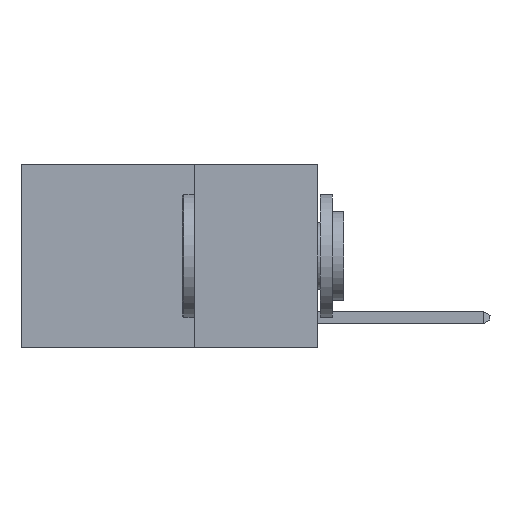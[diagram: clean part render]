
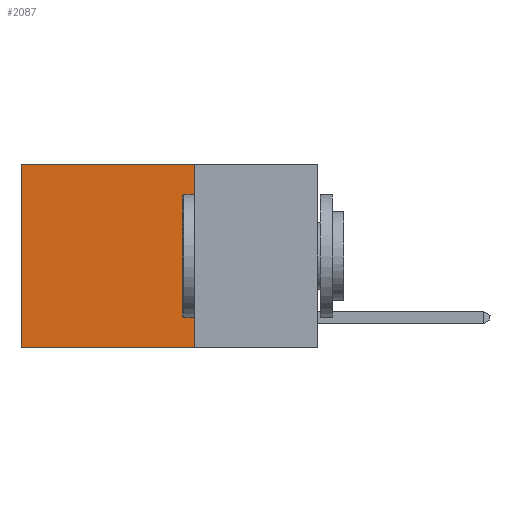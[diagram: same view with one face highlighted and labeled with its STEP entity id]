
A CAD part, left-side view. The second image highlights one B-rep face of the part: STEP entity #2087.
In plain terms, the highlighted planar face has unit normal (-1, 0, 0).
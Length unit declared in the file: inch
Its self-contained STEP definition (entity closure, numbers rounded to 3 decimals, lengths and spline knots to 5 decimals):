
#336 = EDGE_CURVE ( 'NONE', #4194, #12031, #13688, .T. ) ;
#573 = CARTESIAN_POINT ( 'NONE',  ( 0.2625, 0.6, 0. ) ) ;
#1482 = LINE ( 'NONE', #6404, #11278 ) ;
#1989 = VERTEX_POINT ( 'NONE', #8276 ) ;
#1996 = EDGE_CURVE ( 'NONE', #1989, #13666, #3204, .T. ) ;
#2087 = ADVANCED_FACE ( 'NONE', ( #5139 ), #3523, .F. ) ;
#2537 = VECTOR ( 'NONE', #7542, 39.37008 ) ;
#3204 = LINE ( 'NONE', #5644, #10374 ) ;
#3414 = CARTESIAN_POINT ( 'NONE',  ( 0.2625, 0.6, 0. ) ) ;
#3523 = PLANE ( 'NONE',  #10117 ) ;
#3543 = DIRECTION ( 'NONE',  ( 0., 1., 0. ) ) ;
#3694 = CARTESIAN_POINT ( 'NONE',  ( 0.2625, 0.25, 0. ) ) ;
#3885 = EDGE_LOOP ( 'NONE', ( #9423, #12779, #8823, #8395 ) ) ;
#4194 = VERTEX_POINT ( 'NONE', #3414 ) ;
#5139 = FACE_OUTER_BOUND ( 'NONE', #3885, .T. ) ;
#5644 = CARTESIAN_POINT ( 'NONE',  ( 0.2625, 0.25, 0. ) ) ;
#5944 = DIRECTION ( 'NONE',  ( 0., 0., -1. ) ) ;
#6336 = DIRECTION ( 'NONE',  ( 1., 0., 0. ) ) ;
#6404 = CARTESIAN_POINT ( 'NONE',  ( 0.2625, 0.25, 0. ) ) ;
#6932 = CARTESIAN_POINT ( 'NONE',  ( 0.2625, 0.25, -0.37 ) ) ;
#7205 = EDGE_CURVE ( 'NONE', #1989, #4194, #1482, .T. ) ;
#7260 = CARTESIAN_POINT ( 'NONE',  ( 0.2625, 0.25, -0.37 ) ) ;
#7480 = CARTESIAN_POINT ( 'NONE',  ( 0.2625, 0.6, -0.37 ) ) ;
#7542 = DIRECTION ( 'NONE',  ( 0., 0., -1. ) ) ;
#8276 = CARTESIAN_POINT ( 'NONE',  ( 0.2625, 0.25, 0. ) ) ;
#8291 = EDGE_CURVE ( 'NONE', #13666, #12031, #14695, .T. ) ;
#8395 = ORIENTED_EDGE ( 'NONE', *, *, #7205, .T. ) ;
#8823 = ORIENTED_EDGE ( 'NONE', *, *, #1996, .F. ) ;
#9423 = ORIENTED_EDGE ( 'NONE', *, *, #336, .T. ) ;
#10117 = AXIS2_PLACEMENT_3D ( 'NONE', #3694, #6336, #12178 ) ;
#10374 = VECTOR ( 'NONE', #5944, 39.37008 ) ;
#11278 = VECTOR ( 'NONE', #11345, 39.37008 ) ;
#11345 = DIRECTION ( 'NONE',  ( 0., 1., 0. ) ) ;
#12031 = VERTEX_POINT ( 'NONE', #7480 ) ;
#12178 = DIRECTION ( 'NONE',  ( 0., 0., -1. ) ) ;
#12779 = ORIENTED_EDGE ( 'NONE', *, *, #8291, .F. ) ;
#13666 = VERTEX_POINT ( 'NONE', #6932 ) ;
#13688 = LINE ( 'NONE', #573, #2537 ) ;
#13864 = VECTOR ( 'NONE', #3543, 39.37008 ) ;
#14695 = LINE ( 'NONE', #7260, #13864 ) ;
